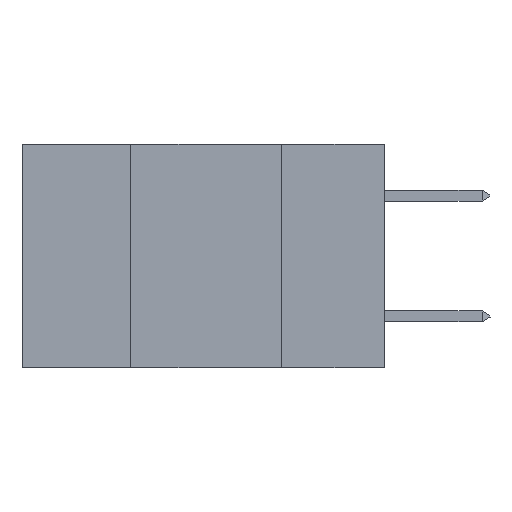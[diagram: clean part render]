
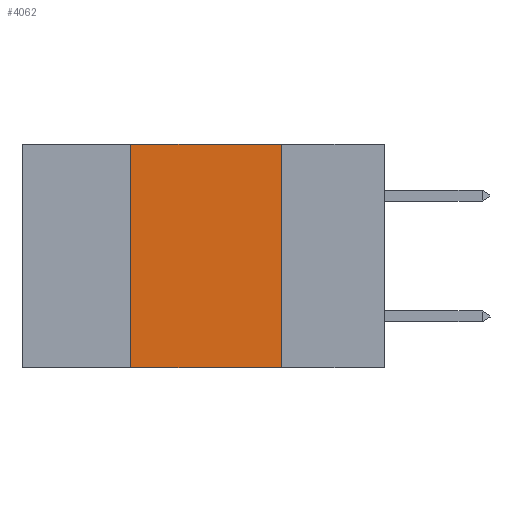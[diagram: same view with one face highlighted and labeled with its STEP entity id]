
A CAD part, left-side view. The second image highlights one B-rep face of the part: STEP entity #4062.
In plain terms, the highlighted planar face has unit normal (-1, 0, 0).
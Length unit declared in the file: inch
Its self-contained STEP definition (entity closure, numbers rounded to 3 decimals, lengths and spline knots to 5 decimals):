
#391 = PLANE ( 'NONE',  #18715 ) ;
#723 = VERTEX_POINT ( 'NONE', #4094 ) ;
#1186 = EDGE_CURVE ( 'NONE', #14471, #7868, #6057, .T. ) ;
#2191 = EDGE_LOOP ( 'NONE', ( #15825, #17214, #16787, #14879 ) ) ;
#2945 = LINE ( 'NONE', #11018, #15619 ) ;
#3985 = DIRECTION ( 'NONE',  ( 0., 0., -1. ) ) ;
#4062 = ADVANCED_FACE ( 'NONE', ( #19248 ), #391, .F. ) ;
#4094 = CARTESIAN_POINT ( 'NONE',  ( 0., 0.17, -0.37 ) ) ;
#5074 = DIRECTION ( 'NONE',  ( 0., 0., -1. ) ) ;
#5606 = EDGE_CURVE ( 'NONE', #6135, #723, #19679, .T. ) ;
#6057 = LINE ( 'NONE', #15832, #17505 ) ;
#6135 = VERTEX_POINT ( 'NONE', #13158 ) ;
#6160 = DIRECTION ( 'NONE',  ( 0., -1., 0. ) ) ;
#7868 = VERTEX_POINT ( 'NONE', #16654 ) ;
#9444 = EDGE_CURVE ( 'NONE', #14471, #723, #18582, .T. ) ;
#10965 = VECTOR ( 'NONE', #17641, 39.37008 ) ;
#11018 = CARTESIAN_POINT ( 'NONE',  ( 0., 0.6, 0. ) ) ;
#11333 = CARTESIAN_POINT ( 'NONE',  ( 0., 0.42, -0.37 ) ) ;
#12118 = CARTESIAN_POINT ( 'NONE',  ( 0., 0.17, 0. ) ) ;
#12213 = CARTESIAN_POINT ( 'NONE',  ( 0., 0.6, 0. ) ) ;
#13158 = CARTESIAN_POINT ( 'NONE',  ( 0., 0.17, 0. ) ) ;
#14373 = CARTESIAN_POINT ( 'NONE',  ( 0., 0.6, -0.37 ) ) ;
#14471 = VERTEX_POINT ( 'NONE', #11333 ) ;
#14879 = ORIENTED_EDGE ( 'NONE', *, *, #9444, .T. ) ;
#15619 = VECTOR ( 'NONE', #6160, 39.37008 ) ;
#15761 = DIRECTION ( 'NONE',  ( 0., 0., 1. ) ) ;
#15825 = ORIENTED_EDGE ( 'NONE', *, *, #5606, .F. ) ;
#15832 = CARTESIAN_POINT ( 'NONE',  ( 0., 0.42, 0. ) ) ;
#16251 = DIRECTION ( 'NONE',  ( 1., 0., 0. ) ) ;
#16654 = CARTESIAN_POINT ( 'NONE',  ( 0., 0.42, 0. ) ) ;
#16787 = ORIENTED_EDGE ( 'NONE', *, *, #1186, .F. ) ;
#17214 = ORIENTED_EDGE ( 'NONE', *, *, #19964, .F. ) ;
#17505 = VECTOR ( 'NONE', #15761, 39.37008 ) ;
#17641 = DIRECTION ( 'NONE',  ( 0., -1., 0. ) ) ;
#18582 = LINE ( 'NONE', #14373, #10965 ) ;
#18715 = AXIS2_PLACEMENT_3D ( 'NONE', #12213, #16251, #5074 ) ;
#19248 = FACE_OUTER_BOUND ( 'NONE', #2191, .T. ) ;
#19679 = LINE ( 'NONE', #12118, #19929 ) ;
#19929 = VECTOR ( 'NONE', #3985, 39.37008 ) ;
#19964 = EDGE_CURVE ( 'NONE', #7868, #6135, #2945, .T. ) ;
